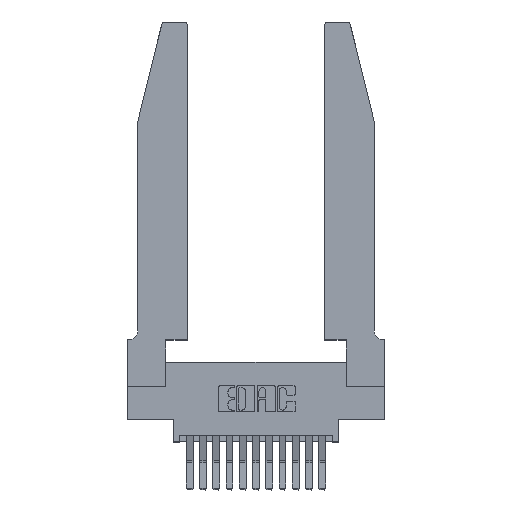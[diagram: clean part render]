
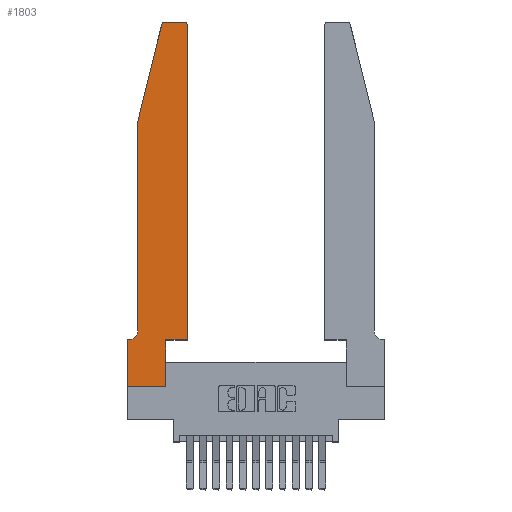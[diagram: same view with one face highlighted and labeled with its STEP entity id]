
A CAD part, top view. The second image highlights one B-rep face of the part: STEP entity #1803.
In plain terms, the highlighted planar face has unit normal (0, 0, 1).
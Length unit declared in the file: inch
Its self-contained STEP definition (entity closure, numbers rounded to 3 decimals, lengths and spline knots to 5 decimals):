
#406 = CARTESIAN_POINT ( 'NONE',  ( 0.0755, 2., 0.37 ) ) ;
#685 = VERTEX_POINT ( 'NONE', #12989 ) ;
#900 = CARTESIAN_POINT ( 'NONE',  ( 0., 0., 0.37 ) ) ;
#930 = VECTOR ( 'NONE', #12715, 39.37008 ) ;
#994 = VECTOR ( 'NONE', #14868, 39.37008 ) ;
#1290 = LINE ( 'NONE', #900, #11455 ) ;
#1676 = CARTESIAN_POINT ( 'NONE',  ( 0.0055, 0.35, 0.37 ) ) ;
#1774 = VERTEX_POINT ( 'NONE', #4513 ) ;
#1803 = ADVANCED_FACE ( 'NONE', ( #6516 ), #2885, .T. ) ;
#2239 = VERTEX_POINT ( 'NONE', #5899 ) ;
#2252 = DIRECTION ( 'NONE',  ( 0., 0., -1. ) ) ;
#2342 = DIRECTION ( 'NONE',  ( 0., 0., 1. ) ) ;
#2414 = DIRECTION ( 'NONE',  ( 1., 0., 0. ) ) ;
#2449 = VERTEX_POINT ( 'NONE', #5527 ) ;
#2640 = CARTESIAN_POINT ( 'NONE',  ( 0.284, 2.75, 0.37 ) ) ;
#2802 = LINE ( 'NONE', #12505, #6107 ) ;
#2885 = PLANE ( 'NONE',  #7174 ) ;
#2949 = ORIENTED_EDGE ( 'NONE', *, *, #11744, .T. ) ;
#3148 = EDGE_CURVE ( 'NONE', #1774, #685, #6268, .T. ) ;
#3415 = DIRECTION ( 'NONE',  ( 1., 0., 0. ) ) ;
#3601 = ORIENTED_EDGE ( 'NONE', *, *, #10675, .T. ) ;
#3649 = DIRECTION ( 'NONE',  ( -1., 0., 0. ) ) ;
#3678 = LINE ( 'NONE', #11526, #14532 ) ;
#3856 = EDGE_CURVE ( 'NONE', #685, #8640, #5722, .T. ) ;
#3893 = AXIS2_PLACEMENT_3D ( 'NONE', #6739, #16195, #8116 ) ;
#4107 = VERTEX_POINT ( 'NONE', #16406 ) ;
#4114 = VECTOR ( 'NONE', #11113, 39.37008 ) ;
#4227 = AXIS2_PLACEMENT_3D ( 'NONE', #6899, #16351, #8266 ) ;
#4370 = CARTESIAN_POINT ( 'NONE',  ( 0.2605, 2.75, 0.37 ) ) ;
#4504 = CARTESIAN_POINT ( 'NONE',  ( 0.4505, 2.72, 0.37 ) ) ;
#4513 = CARTESIAN_POINT ( 'NONE',  ( 0.0755, 2., 0.37 ) ) ;
#4527 = CIRCLE ( 'NONE', #3893, 0.03 ) ;
#4539 = LINE ( 'NONE', #4370, #4114 ) ;
#4693 = EDGE_CURVE ( 'NONE', #4107, #14599, #11624, .T. ) ;
#4737 = ORIENTED_EDGE ( 'NONE', *, *, #13761, .T. ) ;
#4821 = LINE ( 'NONE', #15321, #930 ) ;
#4972 = DIRECTION ( 'NONE',  ( 1., 0., 0. ) ) ;
#5260 = VERTEX_POINT ( 'NONE', #5550 ) ;
#5442 = LINE ( 'NONE', #17192, #8211 ) ;
#5527 = CARTESIAN_POINT ( 'NONE',  ( 0.2865, 0., 0.37 ) ) ;
#5550 = CARTESIAN_POINT ( 'NONE',  ( 0.4205, 2.75, 0.37 ) ) ;
#5647 = ORIENTED_EDGE ( 'NONE', *, *, #7264, .T. ) ;
#5722 = CIRCLE ( 'NONE', #13637, 0.07 ) ;
#5828 = DIRECTION ( 'NONE',  ( 0., -1., 0. ) ) ;
#5899 = CARTESIAN_POINT ( 'NONE',  ( 0., 0., 0.37 ) ) ;
#6044 = EDGE_CURVE ( 'NONE', #16693, #1774, #4821, .T. ) ;
#6097 = EDGE_LOOP ( 'NONE', ( #16236, #3601, #12172, #16475, #15783, #2949, #8333, #12421, #11642, #5647, #10275, #4737 ) ) ;
#6107 = VECTOR ( 'NONE', #5828, 39.37008 ) ;
#6165 = LINE ( 'NONE', #17456, #12917 ) ;
#6210 = CARTESIAN_POINT ( 'NONE',  ( 0.2865, 0.35, 0.37 ) ) ;
#6268 = LINE ( 'NONE', #406, #16603 ) ;
#6341 = CARTESIAN_POINT ( 'NONE',  ( 0., 0.35, 0.37 ) ) ;
#6516 = FACE_OUTER_BOUND ( 'NONE', #6097, .T. ) ;
#6739 = CARTESIAN_POINT ( 'NONE',  ( 0.4205, 2.72, 0.37 ) ) ;
#6898 = VERTEX_POINT ( 'NONE', #2640 ) ;
#6899 = CARTESIAN_POINT ( 'NONE',  ( 0.284, 2.72, 0.37 ) ) ;
#7174 = AXIS2_PLACEMENT_3D ( 'NONE', #6341, #2342, #4972 ) ;
#7264 = EDGE_CURVE ( 'NONE', #12667, #4107, #3678, .T. ) ;
#7643 = EDGE_CURVE ( 'NONE', #5260, #6898, #4539, .T. ) ;
#8048 = CARTESIAN_POINT ( 'NONE',  ( 0., 0.35, 0.37 ) ) ;
#8116 = DIRECTION ( 'NONE',  ( 1., 0., 0. ) ) ;
#8131 = CARTESIAN_POINT ( 'NONE',  ( 0.25487, 2.72718, 0.37 ) ) ;
#8211 = VECTOR ( 'NONE', #3649, 39.37008 ) ;
#8265 = VERTEX_POINT ( 'NONE', #8048 ) ;
#8266 = DIRECTION ( 'NONE',  ( 1., 0., 0. ) ) ;
#8333 = ORIENTED_EDGE ( 'NONE', *, *, #11457, .T. ) ;
#8640 = VERTEX_POINT ( 'NONE', #1676 ) ;
#8854 = DIRECTION ( 'NONE',  ( 0., -1., 0. ) ) ;
#9369 = EDGE_CURVE ( 'NONE', #2239, #2449, #1290, .T. ) ;
#10275 = ORIENTED_EDGE ( 'NONE', *, *, #4693, .T. ) ;
#10511 = CARTESIAN_POINT ( 'NONE',  ( 0.0055, 0.42, 0.37 ) ) ;
#10675 = EDGE_CURVE ( 'NONE', #6898, #16693, #11184, .T. ) ;
#10759 = DIRECTION ( 'NONE',  ( 0., 1., 0. ) ) ;
#11113 = DIRECTION ( 'NONE',  ( -1., 0., 0. ) ) ;
#11184 = CIRCLE ( 'NONE', #4227, 0.03 ) ;
#11455 = VECTOR ( 'NONE', #2414, 39.37008 ) ;
#11457 = EDGE_CURVE ( 'NONE', #8265, #2239, #2802, .T. ) ;
#11526 = CARTESIAN_POINT ( 'NONE',  ( 0.4505, 0.35, 0.37 ) ) ;
#11624 = LINE ( 'NONE', #16168, #994 ) ;
#11642 = ORIENTED_EDGE ( 'NONE', *, *, #16658, .T. ) ;
#11744 = EDGE_CURVE ( 'NONE', #8640, #8265, #5442, .T. ) ;
#11856 = DIRECTION ( 'NONE',  ( -1., 0., 0. ) ) ;
#12172 = ORIENTED_EDGE ( 'NONE', *, *, #6044, .T. ) ;
#12421 = ORIENTED_EDGE ( 'NONE', *, *, #9369, .T. ) ;
#12505 = CARTESIAN_POINT ( 'NONE',  ( 0., 0., 0.37 ) ) ;
#12667 = VERTEX_POINT ( 'NONE', #6210 ) ;
#12715 = DIRECTION ( 'NONE',  ( -0.239, -0.971, 0. ) ) ;
#12917 = VECTOR ( 'NONE', #10759, 39.37008 ) ;
#12989 = CARTESIAN_POINT ( 'NONE',  ( 0.0755, 0.42, 0.37 ) ) ;
#13637 = AXIS2_PLACEMENT_3D ( 'NONE', #10511, #2252, #11856 ) ;
#13761 = EDGE_CURVE ( 'NONE', #14599, #5260, #4527, .T. ) ;
#14532 = VECTOR ( 'NONE', #3415, 39.37008 ) ;
#14599 = VERTEX_POINT ( 'NONE', #4504 ) ;
#14868 = DIRECTION ( 'NONE',  ( 0., 1., 0. ) ) ;
#15321 = CARTESIAN_POINT ( 'NONE',  ( 0.0755, 2., 0.37 ) ) ;
#15783 = ORIENTED_EDGE ( 'NONE', *, *, #3856, .T. ) ;
#16168 = CARTESIAN_POINT ( 'NONE',  ( 0.4505, 0.35, 0.37 ) ) ;
#16195 = DIRECTION ( 'NONE',  ( 0., 0., 1. ) ) ;
#16236 = ORIENTED_EDGE ( 'NONE', *, *, #7643, .T. ) ;
#16351 = DIRECTION ( 'NONE',  ( 0., 0., 1. ) ) ;
#16406 = CARTESIAN_POINT ( 'NONE',  ( 0.4505, 0.35, 0.37 ) ) ;
#16475 = ORIENTED_EDGE ( 'NONE', *, *, #3148, .T. ) ;
#16603 = VECTOR ( 'NONE', #8854, 39.37008 ) ;
#16658 = EDGE_CURVE ( 'NONE', #2449, #12667, #6165, .T. ) ;
#16693 = VERTEX_POINT ( 'NONE', #8131 ) ;
#17192 = CARTESIAN_POINT ( 'NONE',  ( 0.0755, 0.35, 0.37 ) ) ;
#17456 = CARTESIAN_POINT ( 'NONE',  ( 0.2865, 0.35, 0.37 ) ) ;
